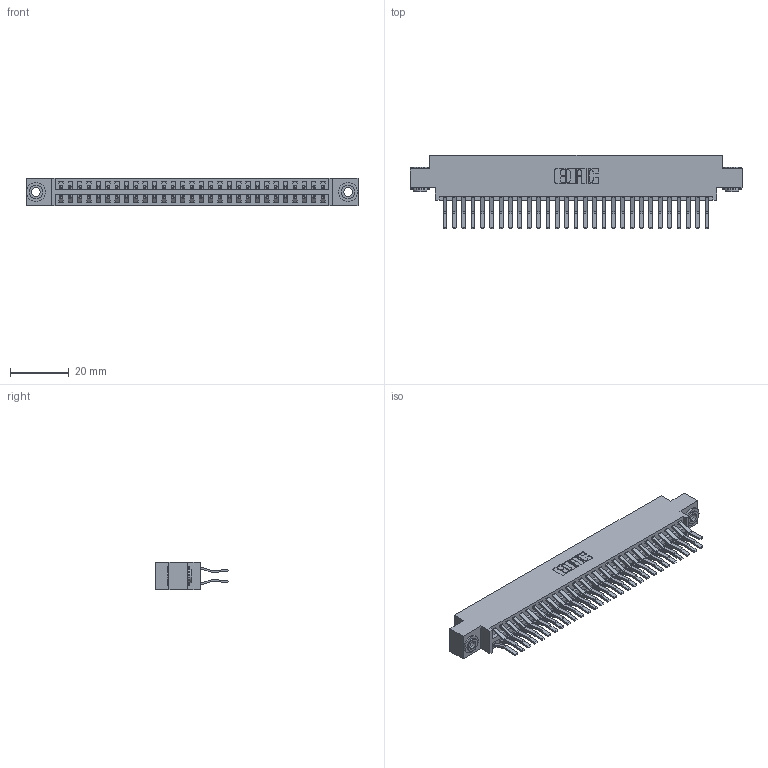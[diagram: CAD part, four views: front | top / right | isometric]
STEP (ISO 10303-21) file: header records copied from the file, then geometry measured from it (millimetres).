
FILE_DESCRIPTION (( 'STEP AP203' ), '1' );
FILE_NAME ('396-058-560-803.STEP', '2019-11-02T08:49:19', ( '' ), ( '' ), 'SwSTEP 2.0', 'SolidWorks 2016', '' );
FILE_SCHEMA (( 'CONFIG_CONTROL_DESIGN' ));
Length unit declared in the file: inch
Products named in the file (4): 346 Part_0.170 Offset - 0.156 Dia-TH; 345-292-001_560 Tail; 345-250-002_345-250-002-102; 396-058-560-803
Assembly tree (61 placements, depth 2):
  396-058-560-803
    346 Part_0.170 Offset - 0.156 Dia-TH
    345-292-001_560 Tail  x58
    345-250-002_345-250-002-102  x2
Bounding box: 112.65 x 24.78 x 9.4 mm (x, y, z)
Volume: 11128.7 mm3; surface area: 16500.8 mm2
Topology: 61 solids, 61 shells, 3296 faces, 9755 edges, 6422 vertices
Faces by surface type: plane 2120, cylinder 1168, cone 8
Entity records: 21546 total; most frequent: CARTESIAN_POINT 3547, ORIENTED_EDGE 3474, DIRECTION 3211, EDGE_CURVE 1737, VECTOR 1461, LINE 1461, VERTEX_POINT 1154, AXIS2_PLACEMENT_3D 875
